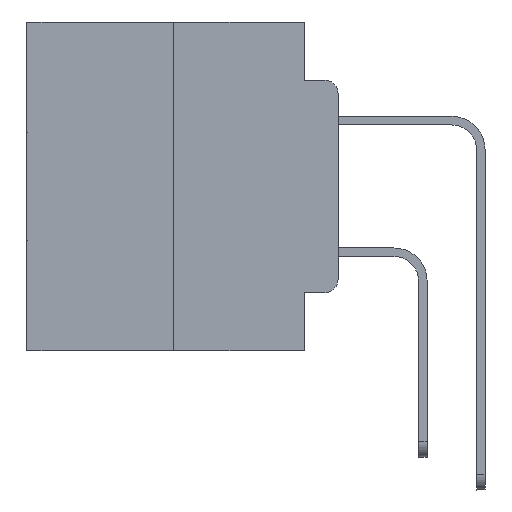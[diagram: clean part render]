
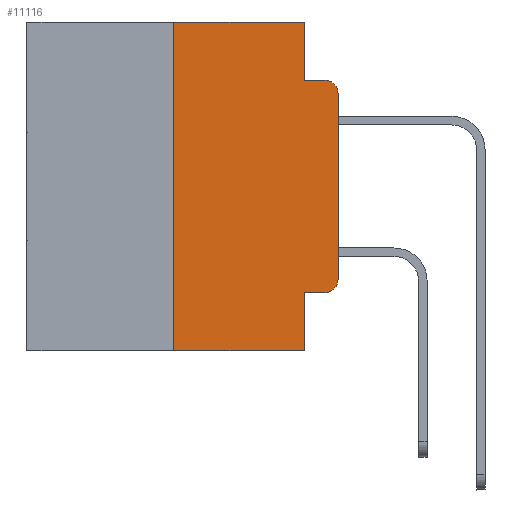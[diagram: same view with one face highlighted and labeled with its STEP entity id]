
A CAD part, left-side view. The second image highlights one B-rep face of the part: STEP entity #11116.
In plain terms, the highlighted planar face has unit normal (-1, 0, 0).
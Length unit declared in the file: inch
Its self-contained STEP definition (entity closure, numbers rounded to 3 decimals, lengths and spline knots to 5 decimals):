
#227 = VERTEX_POINT ( 'NONE', #14588 ) ;
#525 = LINE ( 'NONE', #981, #13747 ) ;
#546 = DIRECTION ( 'NONE',  ( 0., 0., -1. ) ) ;
#981 = CARTESIAN_POINT ( 'NONE',  ( 0., 0.25, 0. ) ) ;
#1133 = VECTOR ( 'NONE', #21510, 39.37008 ) ;
#1513 = CARTESIAN_POINT ( 'NONE',  ( 0., 0.25, -0.5 ) ) ;
#1544 = CARTESIAN_POINT ( 'NONE',  ( 0., 0.473, -0.5 ) ) ;
#1833 = VERTEX_POINT ( 'NONE', #5754 ) ;
#2039 = VERTEX_POINT ( 'NONE', #25961 ) ;
#2444 = ORIENTED_EDGE ( 'NONE', *, *, #6402, .T. ) ;
#2690 = PLANE ( 'NONE',  #29183 ) ;
#3114 = CARTESIAN_POINT ( 'NONE',  ( 0., 0.051, -0.4115 ) ) ;
#3141 = CARTESIAN_POINT ( 'NONE',  ( 0., 0.473, 0. ) ) ;
#3268 = VERTEX_POINT ( 'NONE', #20066 ) ;
#3338 = ORIENTED_EDGE ( 'NONE', *, *, #7948, .F. ) ;
#3394 = LINE ( 'NONE', #1544, #17372 ) ;
#4377 = ORIENTED_EDGE ( 'NONE', *, *, #18313, .F. ) ;
#4442 = LINE ( 'NONE', #6403, #10174 ) ;
#4947 = DIRECTION ( 'NONE',  ( 0., 0., -1. ) ) ;
#5128 = ORIENTED_EDGE ( 'NONE', *, *, #21531, .T. ) ;
#5137 = CARTESIAN_POINT ( 'NONE',  ( 0., 0., 0. ) ) ;
#5589 = CIRCLE ( 'NONE', #19184, 0.02 ) ;
#5754 = CARTESIAN_POINT ( 'NONE',  ( 0., 0.051, -0.0885 ) ) ;
#5833 = DIRECTION ( 'NONE',  ( 0., 0., 1. ) ) ;
#6402 = EDGE_CURVE ( 'NONE', #10507, #10140, #3394, .T. ) ;
#6403 = CARTESIAN_POINT ( 'NONE',  ( 0., 0.051, 0. ) ) ;
#6578 = VECTOR ( 'NONE', #5833, 39.37008 ) ;
#6750 = VECTOR ( 'NONE', #11566, 39.37008 ) ;
#7508 = LINE ( 'NONE', #3114, #1133 ) ;
#7908 = EDGE_CURVE ( 'NONE', #11370, #1833, #11409, .T. ) ;
#7948 = EDGE_CURVE ( 'NONE', #19837, #10140, #4442, .T. ) ;
#8039 = CARTESIAN_POINT ( 'NONE',  ( 0., 0.25, 0. ) ) ;
#8463 = VERTEX_POINT ( 'NONE', #16838 ) ;
#8504 = VECTOR ( 'NONE', #13257, 39.37008 ) ;
#8986 = CARTESIAN_POINT ( 'NONE',  ( 0., 0.051, 0. ) ) ;
#8997 = VERTEX_POINT ( 'NONE', #8039 ) ;
#9138 = DIRECTION ( 'NONE',  ( 0., 0., -1. ) ) ;
#10140 = VERTEX_POINT ( 'NONE', #11407 ) ;
#10174 = VECTOR ( 'NONE', #9138, 39.37008 ) ;
#10507 = VERTEX_POINT ( 'NONE', #1513 ) ;
#11116 = ADVANCED_FACE ( 'NONE', ( #14217 ), #2690, .F. ) ;
#11370 = VERTEX_POINT ( 'NONE', #22712 ) ;
#11407 = CARTESIAN_POINT ( 'NONE',  ( 0., 0.051, -0.5 ) ) ;
#11409 = LINE ( 'NONE', #8986, #6750 ) ;
#11566 = DIRECTION ( 'NONE',  ( 0., 0., -1. ) ) ;
#12145 = ORIENTED_EDGE ( 'NONE', *, *, #18321, .T. ) ;
#12669 = CARTESIAN_POINT ( 'NONE',  ( 0., 0.051, -0.0885 ) ) ;
#13257 = DIRECTION ( 'NONE',  ( 0., -1., 0. ) ) ;
#13410 = LINE ( 'NONE', #24821, #8504 ) ;
#13747 = VECTOR ( 'NONE', #16773, 39.37008 ) ;
#14135 = DIRECTION ( 'NONE',  ( 0., 0., -1. ) ) ;
#14217 = FACE_OUTER_BOUND ( 'NONE', #17807, .T. ) ;
#14588 = CARTESIAN_POINT ( 'NONE',  ( 0., 0.02, -0.4115 ) ) ;
#15198 = CIRCLE ( 'NONE', #24937, 0.02 ) ;
#15672 = CARTESIAN_POINT ( 'NONE',  ( 0., 0.051, -0.4115 ) ) ;
#16429 = EDGE_CURVE ( 'NONE', #2039, #3268, #17369, .T. ) ;
#16773 = DIRECTION ( 'NONE',  ( 0., 0., 1. ) ) ;
#16838 = CARTESIAN_POINT ( 'NONE',  ( 0., 0.02, -0.0885 ) ) ;
#17191 = DIRECTION ( 'NONE',  ( 0., -1., 0. ) ) ;
#17226 = ORIENTED_EDGE ( 'NONE', *, *, #29665, .T. ) ;
#17369 = LINE ( 'NONE', #5137, #6578 ) ;
#17372 = VECTOR ( 'NONE', #17191, 39.37008 ) ;
#17807 = EDGE_LOOP ( 'NONE', ( #19221, #5128, #19324, #23487, #29749, #4377, #2444, #3338, #12145, #17226 ) ) ;
#18310 = DIRECTION ( 'NONE',  ( -1., 0., 0. ) ) ;
#18313 = EDGE_CURVE ( 'NONE', #10507, #8997, #525, .T. ) ;
#18321 = EDGE_CURVE ( 'NONE', #19837, #227, #7508, .T. ) ;
#19184 = AXIS2_PLACEMENT_3D ( 'NONE', #20601, #18310, #4947 ) ;
#19221 = ORIENTED_EDGE ( 'NONE', *, *, #16429, .T. ) ;
#19324 = ORIENTED_EDGE ( 'NONE', *, *, #24350, .F. ) ;
#19518 = DIRECTION ( 'NONE',  ( 0., -1., 0. ) ) ;
#19789 = EDGE_CURVE ( 'NONE', #8997, #11370, #13410, .T. ) ;
#19837 = VERTEX_POINT ( 'NONE', #15672 ) ;
#20066 = CARTESIAN_POINT ( 'NONE',  ( 0., 0., -0.1085 ) ) ;
#20601 = CARTESIAN_POINT ( 'NONE',  ( 0., 0.02, -0.1085 ) ) ;
#20846 = DIRECTION ( 'NONE',  ( -1., 0., 0. ) ) ;
#21510 = DIRECTION ( 'NONE',  ( 0., -1., 0. ) ) ;
#21531 = EDGE_CURVE ( 'NONE', #3268, #8463, #5589, .T. ) ;
#21823 = LINE ( 'NONE', #12669, #27105 ) ;
#22712 = CARTESIAN_POINT ( 'NONE',  ( 0., 0.051, 0. ) ) ;
#22961 = CARTESIAN_POINT ( 'NONE',  ( 0., 0.02, -0.3915 ) ) ;
#23487 = ORIENTED_EDGE ( 'NONE', *, *, #7908, .F. ) ;
#24350 = EDGE_CURVE ( 'NONE', #1833, #8463, #21823, .T. ) ;
#24821 = CARTESIAN_POINT ( 'NONE',  ( 0., 0.473, 0. ) ) ;
#24937 = AXIS2_PLACEMENT_3D ( 'NONE', #22961, #20846, #14135 ) ;
#25801 = DIRECTION ( 'NONE',  ( 1., 0., 0. ) ) ;
#25961 = CARTESIAN_POINT ( 'NONE',  ( 0., 0., -0.3915 ) ) ;
#27105 = VECTOR ( 'NONE', #19518, 39.37008 ) ;
#29183 = AXIS2_PLACEMENT_3D ( 'NONE', #3141, #25801, #546 ) ;
#29665 = EDGE_CURVE ( 'NONE', #227, #2039, #15198, .T. ) ;
#29749 = ORIENTED_EDGE ( 'NONE', *, *, #19789, .F. ) ;
